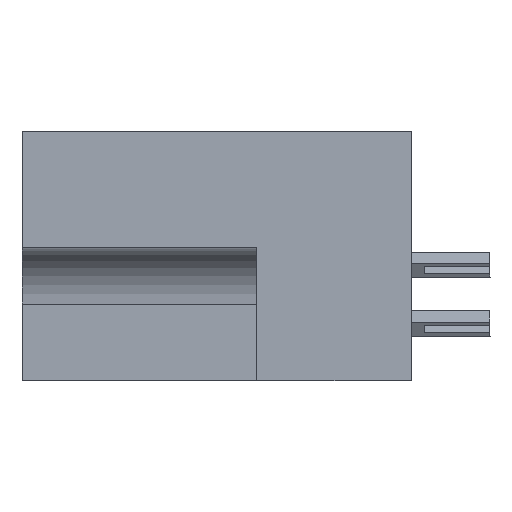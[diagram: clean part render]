
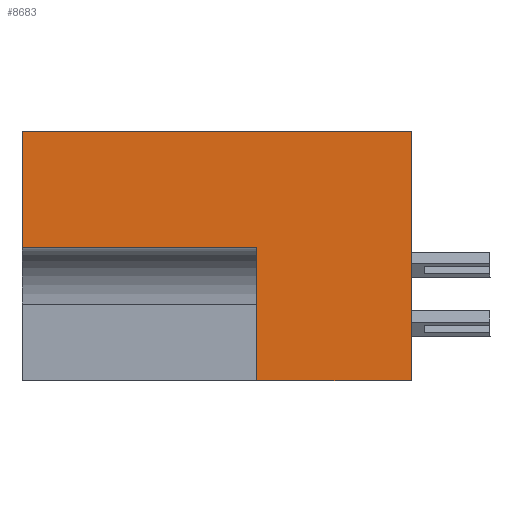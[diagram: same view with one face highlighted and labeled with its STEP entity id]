
A CAD part, left-side view. The second image highlights one B-rep face of the part: STEP entity #8683.
In plain terms, the highlighted planar face has unit normal (-1, 0, 0).
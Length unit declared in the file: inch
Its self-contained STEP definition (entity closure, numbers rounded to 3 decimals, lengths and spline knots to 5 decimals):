
#18 = CARTESIAN_POINT ( 'NONE',  ( 0., 0.453, -0.531 ) ) ;
#183 = LINE ( 'NONE', #13357, #4837 ) ;
#339 = LINE ( 'NONE', #7280, #15272 ) ;
#487 = ORIENTED_EDGE ( 'NONE', *, *, #6970, .T. ) ;
#882 = EDGE_CURVE ( 'NONE', #8735, #7272, #183, .T. ) ;
#1219 = VECTOR ( 'NONE', #2361, 39.37008 ) ;
#1287 = VECTOR ( 'NONE', #11008, 39.37008 ) ;
#1787 = LINE ( 'NONE', #18, #1219 ) ;
#2361 = DIRECTION ( 'NONE',  ( 0., -1., 0. ) ) ;
#2779 = VERTEX_POINT ( 'NONE', #12069 ) ;
#3006 = DIRECTION ( 'NONE',  ( 1., 0., 0. ) ) ;
#3028 = DIRECTION ( 'NONE',  ( 0., -1., 0. ) ) ;
#3721 = VERTEX_POINT ( 'NONE', #5359 ) ;
#4014 = CARTESIAN_POINT ( 'NONE',  ( 0., 0.453, 0. ) ) ;
#4223 = PLANE ( 'NONE',  #10360 ) ;
#4520 = DIRECTION ( 'NONE',  ( 0., 0., 1. ) ) ;
#4768 = EDGE_CURVE ( 'NONE', #2779, #6934, #14884, .T. ) ;
#4837 = VECTOR ( 'NONE', #8449, 39.37008 ) ;
#4973 = ORIENTED_EDGE ( 'NONE', *, *, #882, .T. ) ;
#5039 = VERTEX_POINT ( 'NONE', #15376 ) ;
#5328 = CARTESIAN_POINT ( 'NONE',  ( 0., 0., -0.531 ) ) ;
#5359 = CARTESIAN_POINT ( 'NONE',  ( 0., 0.828, 0. ) ) ;
#6934 = VERTEX_POINT ( 'NONE', #12112 ) ;
#6970 = EDGE_CURVE ( 'NONE', #5039, #8735, #1787, .T. ) ;
#7163 = CARTESIAN_POINT ( 'NONE',  ( 0., 0.328, -0.531 ) ) ;
#7272 = VERTEX_POINT ( 'NONE', #14384 ) ;
#7280 = CARTESIAN_POINT ( 'NONE',  ( 0., 0.828, 0. ) ) ;
#7845 = ORIENTED_EDGE ( 'NONE', *, *, #13802, .F. ) ;
#8449 = DIRECTION ( 'NONE',  ( 0., 0., 1. ) ) ;
#8674 = DIRECTION ( 'NONE',  ( 0., 0., 1. ) ) ;
#8683 = ADVANCED_FACE ( 'NONE', ( #16098 ), #4223, .F. ) ;
#8735 = VERTEX_POINT ( 'NONE', #5328 ) ;
#9898 = EDGE_LOOP ( 'NONE', ( #7845, #14796, #10667, #487, #4973, #14022 ) ) ;
#10360 = AXIS2_PLACEMENT_3D ( 'NONE', #4014, #3006, #14108 ) ;
#10667 = ORIENTED_EDGE ( 'NONE', *, *, #10900, .F. ) ;
#10900 = EDGE_CURVE ( 'NONE', #5039, #2779, #13644, .T. ) ;
#11008 = DIRECTION ( 'NONE',  ( 0., 1., 0. ) ) ;
#12069 = CARTESIAN_POINT ( 'NONE',  ( 0., 0.328, -0.248 ) ) ;
#12112 = CARTESIAN_POINT ( 'NONE',  ( 0., 0.828, -0.248 ) ) ;
#12259 = VECTOR ( 'NONE', #4520, 39.37008 ) ;
#12843 = CARTESIAN_POINT ( 'NONE',  ( 0., 0.453, 0. ) ) ;
#13345 = CARTESIAN_POINT ( 'NONE',  ( 0., 0.328, -0.248 ) ) ;
#13357 = CARTESIAN_POINT ( 'NONE',  ( 0., 0., 0. ) ) ;
#13644 = LINE ( 'NONE', #7163, #12259 ) ;
#13802 = EDGE_CURVE ( 'NONE', #6934, #3721, #339, .T. ) ;
#14022 = ORIENTED_EDGE ( 'NONE', *, *, #15513, .F. ) ;
#14035 = LINE ( 'NONE', #12843, #14825 ) ;
#14108 = DIRECTION ( 'NONE',  ( 0., 0., -1. ) ) ;
#14384 = CARTESIAN_POINT ( 'NONE',  ( 0., 0., 0. ) ) ;
#14796 = ORIENTED_EDGE ( 'NONE', *, *, #4768, .F. ) ;
#14825 = VECTOR ( 'NONE', #3028, 39.37008 ) ;
#14884 = LINE ( 'NONE', #13345, #1287 ) ;
#15272 = VECTOR ( 'NONE', #8674, 39.37008 ) ;
#15376 = CARTESIAN_POINT ( 'NONE',  ( 0., 0.328, -0.531 ) ) ;
#15513 = EDGE_CURVE ( 'NONE', #3721, #7272, #14035, .T. ) ;
#16098 = FACE_OUTER_BOUND ( 'NONE', #9898, .T. ) ;
